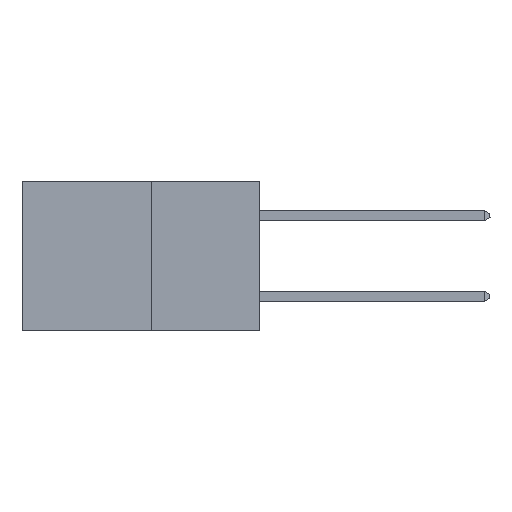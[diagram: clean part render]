
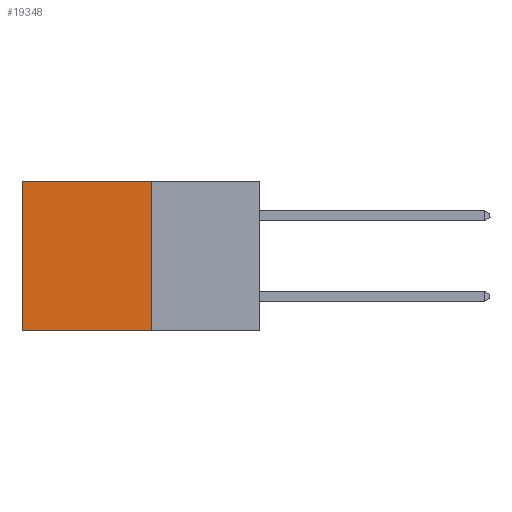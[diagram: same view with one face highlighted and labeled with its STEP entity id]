
A CAD part, left-side view. The second image highlights one B-rep face of the part: STEP entity #19348.
In plain terms, the highlighted planar face has unit normal (-1, 0, 0).
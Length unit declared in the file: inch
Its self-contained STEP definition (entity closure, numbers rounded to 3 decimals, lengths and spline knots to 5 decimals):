
#104 = DIRECTION ( 'NONE',  ( 0., 0., -1. ) ) ;
#403 = CARTESIAN_POINT ( 'NONE',  ( 0.277, 0.27, 0. ) ) ;
#409 = PLANE ( 'NONE',  #18285 ) ;
#831 = LINE ( 'NONE', #3952, #17150 ) ;
#1498 = EDGE_CURVE ( 'NONE', #6764, #11878, #831, .T. ) ;
#1608 = CARTESIAN_POINT ( 'NONE',  ( 0.277, 0.27, 0. ) ) ;
#2660 = ORIENTED_EDGE ( 'NONE', *, *, #14243, .F. ) ;
#3824 = ORIENTED_EDGE ( 'NONE', *, *, #5213, .T. ) ;
#3937 = DIRECTION ( 'NONE',  ( 0., 0., -1. ) ) ;
#3952 = CARTESIAN_POINT ( 'NONE',  ( 0.277, 0.59, -0.37 ) ) ;
#4092 = DIRECTION ( 'NONE',  ( 0., 0., -1. ) ) ;
#4598 = CARTESIAN_POINT ( 'NONE',  ( 0.277, 0.59, -0.37 ) ) ;
#5213 = EDGE_CURVE ( 'NONE', #6699, #6764, #19112, .T. ) ;
#5439 = LINE ( 'NONE', #7688, #19939 ) ;
#5603 = ORIENTED_EDGE ( 'NONE', *, *, #16885, .F. ) ;
#5685 = CARTESIAN_POINT ( 'NONE',  ( 0.277, 0.59, 0. ) ) ;
#6699 = VERTEX_POINT ( 'NONE', #403 ) ;
#6764 = VERTEX_POINT ( 'NONE', #5685 ) ;
#7554 = DIRECTION ( 'NONE',  ( 0., 1., 0. ) ) ;
#7688 = CARTESIAN_POINT ( 'NONE',  ( 0.277, 0.27, -0.37 ) ) ;
#8101 = EDGE_LOOP ( 'NONE', ( #9191, #2660, #5603, #3824 ) ) ;
#8377 = LINE ( 'NONE', #11301, #11998 ) ;
#9191 = ORIENTED_EDGE ( 'NONE', *, *, #1498, .T. ) ;
#11301 = CARTESIAN_POINT ( 'NONE',  ( 0.277, 0.27, -0.37 ) ) ;
#11474 = VERTEX_POINT ( 'NONE', #14044 ) ;
#11568 = CARTESIAN_POINT ( 'NONE',  ( 0.277, 0.27, -0.37 ) ) ;
#11878 = VERTEX_POINT ( 'NONE', #4598 ) ;
#11998 = VECTOR ( 'NONE', #104, 39.37008 ) ;
#12507 = DIRECTION ( 'NONE',  ( 0., 1., 0. ) ) ;
#12790 = FACE_OUTER_BOUND ( 'NONE', #8101, .T. ) ;
#13463 = DIRECTION ( 'NONE',  ( 1., 0., 0. ) ) ;
#14044 = CARTESIAN_POINT ( 'NONE',  ( 0.277, 0.27, -0.37 ) ) ;
#14243 = EDGE_CURVE ( 'NONE', #11474, #11878, #5439, .T. ) ;
#15136 = VECTOR ( 'NONE', #12507, 39.37008 ) ;
#16885 = EDGE_CURVE ( 'NONE', #6699, #11474, #8377, .T. ) ;
#17150 = VECTOR ( 'NONE', #4092, 39.37008 ) ;
#18285 = AXIS2_PLACEMENT_3D ( 'NONE', #11568, #13463, #3937 ) ;
#19112 = LINE ( 'NONE', #1608, #15136 ) ;
#19348 = ADVANCED_FACE ( 'NONE', ( #12790 ), #409, .F. ) ;
#19939 = VECTOR ( 'NONE', #7554, 39.37008 ) ;
